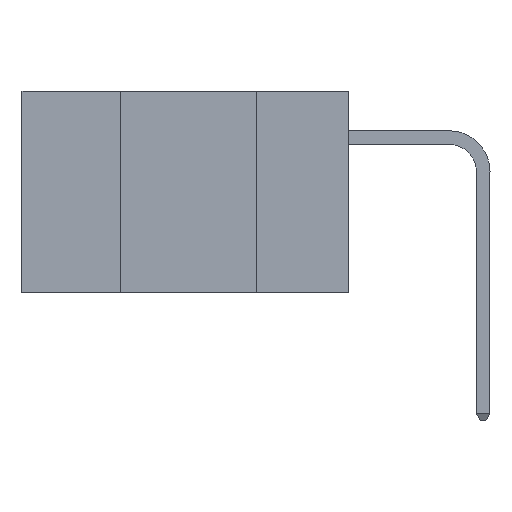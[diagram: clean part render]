
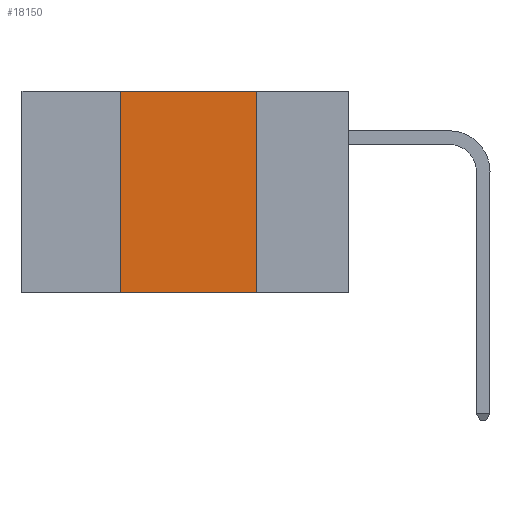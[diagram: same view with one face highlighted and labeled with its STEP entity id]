
A CAD part, left-side view. The second image highlights one B-rep face of the part: STEP entity #18150.
In plain terms, the highlighted planar face has unit normal (-1, 0, 0).
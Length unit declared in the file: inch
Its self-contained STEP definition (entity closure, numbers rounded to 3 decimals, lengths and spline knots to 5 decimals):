
#743 = EDGE_CURVE ( 'NONE', #2461, #7740, #29198, .T. ) ;
#2063 = DIRECTION ( 'NONE',  ( 0., 0., -1. ) ) ;
#2461 = VERTEX_POINT ( 'NONE', #17191 ) ;
#4595 = FACE_OUTER_BOUND ( 'NONE', #25508, .T. ) ;
#6173 = EDGE_CURVE ( 'NONE', #6855, #7619, #21796, .T. ) ;
#6855 = VERTEX_POINT ( 'NONE', #27041 ) ;
#7088 = CARTESIAN_POINT ( 'NONE',  ( 0., 0.6, 0. ) ) ;
#7619 = VERTEX_POINT ( 'NONE', #15231 ) ;
#7640 = VECTOR ( 'NONE', #32449, 39.37008 ) ;
#7681 = ORIENTED_EDGE ( 'NONE', *, *, #743, .T. ) ;
#7740 = VERTEX_POINT ( 'NONE', #10667 ) ;
#9695 = PLANE ( 'NONE',  #15924 ) ;
#10667 = CARTESIAN_POINT ( 'NONE',  ( 0., 0.17, -0.37 ) ) ;
#14150 = CARTESIAN_POINT ( 'NONE',  ( 0., 0.6, -0.37 ) ) ;
#14457 = LINE ( 'NONE', #29786, #7640 ) ;
#14467 = ORIENTED_EDGE ( 'NONE', *, *, #32532, .F. ) ;
#15020 = VECTOR ( 'NONE', #27084, 39.37008 ) ;
#15231 = CARTESIAN_POINT ( 'NONE',  ( 0., 0.17, 0. ) ) ;
#15924 = AXIS2_PLACEMENT_3D ( 'NONE', #7088, #17373, #2063 ) ;
#17191 = CARTESIAN_POINT ( 'NONE',  ( 0., 0.42, -0.37 ) ) ;
#17373 = DIRECTION ( 'NONE',  ( 1., 0., 0. ) ) ;
#18150 = ADVANCED_FACE ( 'NONE', ( #4595 ), #9695, .F. ) ;
#18301 = LINE ( 'NONE', #23698, #24226 ) ;
#19285 = DIRECTION ( 'NONE',  ( 0., -1., 0. ) ) ;
#21796 = LINE ( 'NONE', #24547, #15020 ) ;
#22483 = VECTOR ( 'NONE', #19285, 39.37008 ) ;
#23162 = ORIENTED_EDGE ( 'NONE', *, *, #6173, .F. ) ;
#23698 = CARTESIAN_POINT ( 'NONE',  ( 0., 0.17, 0. ) ) ;
#24226 = VECTOR ( 'NONE', #26236, 39.37008 ) ;
#24547 = CARTESIAN_POINT ( 'NONE',  ( 0., 0.6, 0. ) ) ;
#25508 = EDGE_LOOP ( 'NONE', ( #31273, #23162, #14467, #7681 ) ) ;
#26236 = DIRECTION ( 'NONE',  ( 0., 0., -1. ) ) ;
#27041 = CARTESIAN_POINT ( 'NONE',  ( 0., 0.42, 0. ) ) ;
#27084 = DIRECTION ( 'NONE',  ( 0., -1., 0. ) ) ;
#28487 = EDGE_CURVE ( 'NONE', #7619, #7740, #18301, .T. ) ;
#29198 = LINE ( 'NONE', #14150, #22483 ) ;
#29786 = CARTESIAN_POINT ( 'NONE',  ( 0., 0.42, 0. ) ) ;
#31273 = ORIENTED_EDGE ( 'NONE', *, *, #28487, .F. ) ;
#32449 = DIRECTION ( 'NONE',  ( 0., 0., 1. ) ) ;
#32532 = EDGE_CURVE ( 'NONE', #2461, #6855, #14457, .T. ) ;
